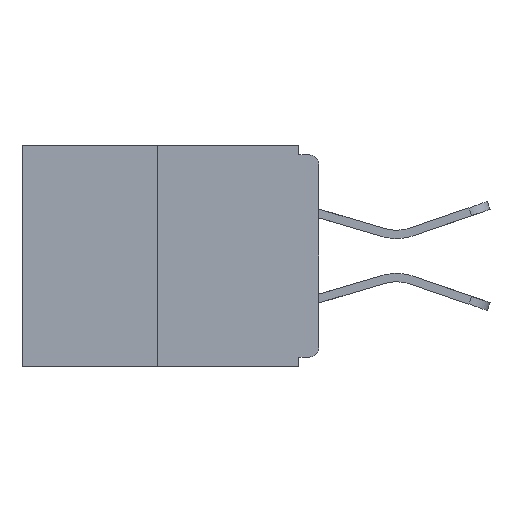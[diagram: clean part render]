
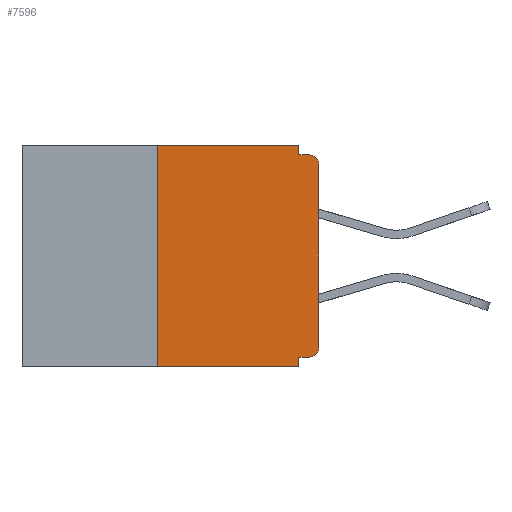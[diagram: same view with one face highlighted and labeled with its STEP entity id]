
A CAD part, left-side view. The second image highlights one B-rep face of the part: STEP entity #7596.
In plain terms, the highlighted planar face has unit normal (-1, 0, 0).
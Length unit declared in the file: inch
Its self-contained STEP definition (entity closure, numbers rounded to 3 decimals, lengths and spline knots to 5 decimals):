
#19 = EDGE_CURVE ( 'NONE', #7283, #6723, #5895, .T. ) ;
#160 = CARTESIAN_POINT ( 'NONE',  ( 0., 0.031, -0.328 ) ) ;
#215 = LINE ( 'NONE', #10378, #8799 ) ;
#337 = CARTESIAN_POINT ( 'NONE',  ( 0., 0.031, 0. ) ) ;
#595 = CIRCLE ( 'NONE', #8139, 0.015 ) ;
#703 = VECTOR ( 'NONE', #11828, 39.37008 ) ;
#1026 = VERTEX_POINT ( 'NONE', #2976 ) ;
#1105 = VECTOR ( 'NONE', #8561, 39.37008 ) ;
#1441 = ORIENTED_EDGE ( 'NONE', *, *, #7563, .F. ) ;
#1443 = ORIENTED_EDGE ( 'NONE', *, *, #19, .F. ) ;
#1579 = VERTEX_POINT ( 'NONE', #8835 ) ;
#1624 = LINE ( 'NONE', #5266, #9518 ) ;
#1729 = EDGE_CURVE ( 'NONE', #6740, #1579, #1624, .T. ) ;
#1757 = DIRECTION ( 'NONE',  ( -1., 0., 0. ) ) ;
#2180 = CARTESIAN_POINT ( 'NONE',  ( 0., 0.031, -0.015 ) ) ;
#2212 = LINE ( 'NONE', #337, #1105 ) ;
#2699 = CARTESIAN_POINT ( 'NONE',  ( 0., 0.015, -0.015 ) ) ;
#2786 = CARTESIAN_POINT ( 'NONE',  ( 0., 0.031, 0. ) ) ;
#2823 = DIRECTION ( 'NONE',  ( 0., 0., -1. ) ) ;
#2914 = PLANE ( 'NONE',  #9574 ) ;
#2924 = VERTEX_POINT ( 'NONE', #2180 ) ;
#2932 = ORIENTED_EDGE ( 'NONE', *, *, #7954, .F. ) ;
#2976 = CARTESIAN_POINT ( 'NONE',  ( 0., 0., -0.03 ) ) ;
#3101 = DIRECTION ( 'NONE',  ( 0., -1., 0. ) ) ;
#3183 = VECTOR ( 'NONE', #6359, 39.37008 ) ;
#3312 = CARTESIAN_POINT ( 'NONE',  ( 0., 0., -0.015 ) ) ;
#3408 = CARTESIAN_POINT ( 'NONE',  ( 0., 0.015, -0.328 ) ) ;
#3555 = EDGE_CURVE ( 'NONE', #10811, #10024, #595, .T. ) ;
#3634 = LINE ( 'NONE', #11747, #3183 ) ;
#4651 = DIRECTION ( 'NONE',  ( 0., 0., -1. ) ) ;
#5105 = CIRCLE ( 'NONE', #7297, 0.015 ) ;
#5126 = CARTESIAN_POINT ( 'NONE',  ( 0., 0., 0. ) ) ;
#5266 = CARTESIAN_POINT ( 'NONE',  ( 0., 0.46, -0.343 ) ) ;
#5278 = CARTESIAN_POINT ( 'NONE',  ( 0., 0., -0.328 ) ) ;
#5424 = CARTESIAN_POINT ( 'NONE',  ( 0., 0.25, -0.343 ) ) ;
#5599 = EDGE_LOOP ( 'NONE', ( #1443, #8293, #5948, #1441, #2932, #8154, #10188, #7040, #7793, #9884 ) ) ;
#5729 = EDGE_CURVE ( 'NONE', #2924, #7141, #8858, .T. ) ;
#5895 = LINE ( 'NONE', #8707, #6442 ) ;
#5923 = DIRECTION ( 'NONE',  ( 0., 0., 1. ) ) ;
#5948 = ORIENTED_EDGE ( 'NONE', *, *, #1729, .T. ) ;
#5959 = CARTESIAN_POINT ( 'NONE',  ( 0., 0.015, -0.03 ) ) ;
#6359 = DIRECTION ( 'NONE',  ( 0., 0., 1. ) ) ;
#6442 = VECTOR ( 'NONE', #3101, 39.37008 ) ;
#6628 = CARTESIAN_POINT ( 'NONE',  ( 0., 0.46, 0. ) ) ;
#6723 = VERTEX_POINT ( 'NONE', #2786 ) ;
#6740 = VERTEX_POINT ( 'NONE', #5424 ) ;
#6881 = VERTEX_POINT ( 'NONE', #160 ) ;
#7040 = ORIENTED_EDGE ( 'NONE', *, *, #8538, .T. ) ;
#7141 = VERTEX_POINT ( 'NONE', #2699 ) ;
#7283 = VERTEX_POINT ( 'NONE', #9744 ) ;
#7297 = AXIS2_PLACEMENT_3D ( 'NONE', #5959, #9660, #4651 ) ;
#7302 = VECTOR ( 'NONE', #9107, 39.37008 ) ;
#7563 = EDGE_CURVE ( 'NONE', #6881, #1579, #215, .T. ) ;
#7596 = ADVANCED_FACE ( 'NONE', ( #11218 ), #2914, .F. ) ;
#7601 = DIRECTION ( 'NONE',  ( 1., 0., 0. ) ) ;
#7707 = LINE ( 'NONE', #5126, #9515 ) ;
#7793 = ORIENTED_EDGE ( 'NONE', *, *, #5729, .F. ) ;
#7954 = EDGE_CURVE ( 'NONE', #10811, #6881, #9893, .T. ) ;
#8139 = AXIS2_PLACEMENT_3D ( 'NONE', #10809, #1757, #11721 ) ;
#8154 = ORIENTED_EDGE ( 'NONE', *, *, #3555, .T. ) ;
#8293 = ORIENTED_EDGE ( 'NONE', *, *, #8498, .F. ) ;
#8498 = EDGE_CURVE ( 'NONE', #6740, #7283, #3634, .T. ) ;
#8538 = EDGE_CURVE ( 'NONE', #1026, #7141, #5105, .T. ) ;
#8561 = DIRECTION ( 'NONE',  ( 0., 0., -1. ) ) ;
#8707 = CARTESIAN_POINT ( 'NONE',  ( 0., 0.46, 0. ) ) ;
#8777 = EDGE_CURVE ( 'NONE', #6723, #2924, #2212, .T. ) ;
#8799 = VECTOR ( 'NONE', #2823, 39.37008 ) ;
#8835 = CARTESIAN_POINT ( 'NONE',  ( 0., 0.031, -0.343 ) ) ;
#8858 = LINE ( 'NONE', #3312, #7302 ) ;
#9002 = DIRECTION ( 'NONE',  ( 0., -1., 0. ) ) ;
#9107 = DIRECTION ( 'NONE',  ( 0., -1., 0. ) ) ;
#9515 = VECTOR ( 'NONE', #5923, 39.37008 ) ;
#9518 = VECTOR ( 'NONE', #9002, 39.37008 ) ;
#9574 = AXIS2_PLACEMENT_3D ( 'NONE', #6628, #7601, #11279 ) ;
#9660 = DIRECTION ( 'NONE',  ( -1., 0., 0. ) ) ;
#9744 = CARTESIAN_POINT ( 'NONE',  ( 0., 0.25, 0. ) ) ;
#9884 = ORIENTED_EDGE ( 'NONE', *, *, #8777, .F. ) ;
#9893 = LINE ( 'NONE', #5278, #703 ) ;
#10024 = VERTEX_POINT ( 'NONE', #11456 ) ;
#10188 = ORIENTED_EDGE ( 'NONE', *, *, #10401, .T. ) ;
#10378 = CARTESIAN_POINT ( 'NONE',  ( 0., 0.031, -0.343 ) ) ;
#10401 = EDGE_CURVE ( 'NONE', #10024, #1026, #7707, .T. ) ;
#10809 = CARTESIAN_POINT ( 'NONE',  ( 0., 0.015, -0.313 ) ) ;
#10811 = VERTEX_POINT ( 'NONE', #3408 ) ;
#11218 = FACE_OUTER_BOUND ( 'NONE', #5599, .T. ) ;
#11279 = DIRECTION ( 'NONE',  ( 0., 0., -1. ) ) ;
#11456 = CARTESIAN_POINT ( 'NONE',  ( 0., 0., -0.313 ) ) ;
#11721 = DIRECTION ( 'NONE',  ( 0., 0., -1. ) ) ;
#11747 = CARTESIAN_POINT ( 'NONE',  ( 0., 0.25, 0. ) ) ;
#11828 = DIRECTION ( 'NONE',  ( 0., 1., 0. ) ) ;
